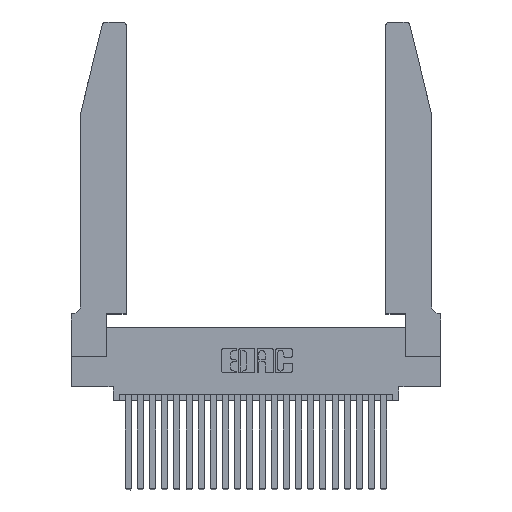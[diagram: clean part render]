
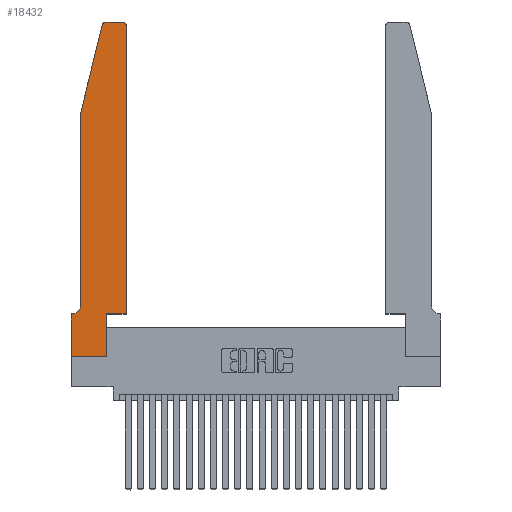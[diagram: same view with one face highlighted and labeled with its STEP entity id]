
A CAD part, top view. The second image highlights one B-rep face of the part: STEP entity #18432.
In plain terms, the highlighted planar face has unit normal (0, 0, 1).
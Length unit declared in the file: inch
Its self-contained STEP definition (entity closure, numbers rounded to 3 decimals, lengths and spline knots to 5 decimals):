
#32 = ORIENTED_EDGE ( 'NONE', *, *, #15384, .T. ) ;
#138 = CARTESIAN_POINT ( 'NONE',  ( 0., 0., 0.37 ) ) ;
#233 = ORIENTED_EDGE ( 'NONE', *, *, #24599, .T. ) ;
#419 = FACE_OUTER_BOUND ( 'NONE', #2256, .T. ) ;
#692 = DIRECTION ( 'NONE',  ( 0., 0., 1. ) ) ;
#938 = CARTESIAN_POINT ( 'NONE',  ( 0.0055, 0.42, 0.37 ) ) ;
#940 = PLANE ( 'NONE',  #18085 ) ;
#1878 = VERTEX_POINT ( 'NONE', #2045 ) ;
#2045 = CARTESIAN_POINT ( 'NONE',  ( 0., 0.35, 0.37 ) ) ;
#2124 = CIRCLE ( 'NONE', #16406, 0.07 ) ;
#2256 = EDGE_LOOP ( 'NONE', ( #233, #3412, #4674, #10498, #32, #19067, #16034, #11661, #19943, #14361, #12221, #11791 ) ) ;
#2813 = DIRECTION ( 'NONE',  ( 1., 0., 0. ) ) ;
#2917 = CARTESIAN_POINT ( 'NONE',  ( 0.2605, 2.75, 0.37 ) ) ;
#2941 = DIRECTION ( 'NONE',  ( 0., 0., 1. ) ) ;
#3209 = VERTEX_POINT ( 'NONE', #20163 ) ;
#3412 = ORIENTED_EDGE ( 'NONE', *, *, #7512, .T. ) ;
#4067 = LINE ( 'NONE', #9989, #20825 ) ;
#4369 = EDGE_CURVE ( 'NONE', #21793, #22872, #14482, .T. ) ;
#4428 = CARTESIAN_POINT ( 'NONE',  ( 0., 0.35, 0.37 ) ) ;
#4674 = ORIENTED_EDGE ( 'NONE', *, *, #23404, .T. ) ;
#4711 = AXIS2_PLACEMENT_3D ( 'NONE', #9152, #7432, #2813 ) ;
#5055 = CARTESIAN_POINT ( 'NONE',  ( 0.25487, 2.72718, 0.37 ) ) ;
#5305 = VERTEX_POINT ( 'NONE', #16759 ) ;
#5505 = LINE ( 'NONE', #2917, #9358 ) ;
#6192 = CARTESIAN_POINT ( 'NONE',  ( 0., 0., 0.37 ) ) ;
#6398 = VERTEX_POINT ( 'NONE', #5055 ) ;
#6475 = VECTOR ( 'NONE', #11939, 39.37008 ) ;
#6639 = CIRCLE ( 'NONE', #4711, 0.03 ) ;
#6866 = CARTESIAN_POINT ( 'NONE',  ( 0.0755, 0.42, 0.37 ) ) ;
#7374 = LINE ( 'NONE', #9487, #13313 ) ;
#7432 = DIRECTION ( 'NONE',  ( 0., 0., 1. ) ) ;
#7512 = EDGE_CURVE ( 'NONE', #3209, #6398, #7634, .T. ) ;
#7634 = CIRCLE ( 'NONE', #19590, 0.03 ) ;
#7831 = CARTESIAN_POINT ( 'NONE',  ( 0.0055, 0.35, 0.37 ) ) ;
#8262 = LINE ( 'NONE', #6192, #6475 ) ;
#8368 = CARTESIAN_POINT ( 'NONE',  ( 0.4505, 0.35, 0.37 ) ) ;
#8622 = CARTESIAN_POINT ( 'NONE',  ( 0.0755, 0.35, 0.37 ) ) ;
#8770 = DIRECTION ( 'NONE',  ( 1., 0., 0. ) ) ;
#8927 = CARTESIAN_POINT ( 'NONE',  ( 0., 0., 0.37 ) ) ;
#9152 = CARTESIAN_POINT ( 'NONE',  ( 0.4205, 2.72, 0.37 ) ) ;
#9326 = VECTOR ( 'NONE', #23130, 39.37008 ) ;
#9358 = VECTOR ( 'NONE', #16198, 39.37008 ) ;
#9365 = LINE ( 'NONE', #8622, #21090 ) ;
#9487 = CARTESIAN_POINT ( 'NONE',  ( 0.2865, 0.35, 0.37 ) ) ;
#9989 = CARTESIAN_POINT ( 'NONE',  ( 0.0755, 2., 0.37 ) ) ;
#10031 = LINE ( 'NONE', #8927, #22606 ) ;
#10269 = VECTOR ( 'NONE', #20962, 39.37008 ) ;
#10498 = ORIENTED_EDGE ( 'NONE', *, *, #4369, .T. ) ;
#11661 = ORIENTED_EDGE ( 'NONE', *, *, #22650, .T. ) ;
#11791 = ORIENTED_EDGE ( 'NONE', *, *, #13497, .T. ) ;
#11823 = EDGE_CURVE ( 'NONE', #5305, #22016, #21979, .T. ) ;
#11939 = DIRECTION ( 'NONE',  ( 1., 0., 0. ) ) ;
#12073 = DIRECTION ( 'NONE',  ( -1., 0., 0. ) ) ;
#12093 = CARTESIAN_POINT ( 'NONE',  ( 0.2865, 0., 0.37 ) ) ;
#12150 = DIRECTION ( 'NONE',  ( 1., 0., 0. ) ) ;
#12221 = ORIENTED_EDGE ( 'NONE', *, *, #18316, .T. ) ;
#12268 = EDGE_CURVE ( 'NONE', #16895, #1878, #9365, .T. ) ;
#12414 = CARTESIAN_POINT ( 'NONE',  ( 0.4505, 2.72, 0.37 ) ) ;
#12465 = DIRECTION ( 'NONE',  ( -1., 0., 0. ) ) ;
#13313 = VECTOR ( 'NONE', #15197, 39.37008 ) ;
#13497 = EDGE_CURVE ( 'NONE', #15955, #16582, #6639, .T. ) ;
#13506 = DIRECTION ( 'NONE',  ( 1., 0., 0. ) ) ;
#13640 = CARTESIAN_POINT ( 'NONE',  ( 0.0755, 2., 0.37 ) ) ;
#13845 = DIRECTION ( 'NONE',  ( -0.239, -0.971, 0. ) ) ;
#14361 = ORIENTED_EDGE ( 'NONE', *, *, #11823, .T. ) ;
#14482 = LINE ( 'NONE', #13640, #10269 ) ;
#15079 = CARTESIAN_POINT ( 'NONE',  ( 0.0755, 2., 0.37 ) ) ;
#15197 = DIRECTION ( 'NONE',  ( 0., 1., 0. ) ) ;
#15384 = EDGE_CURVE ( 'NONE', #22872, #16895, #2124, .T. ) ;
#15689 = VECTOR ( 'NONE', #13506, 39.37008 ) ;
#15864 = DIRECTION ( 'NONE',  ( 0., 0., -1. ) ) ;
#15955 = VERTEX_POINT ( 'NONE', #12414 ) ;
#16034 = ORIENTED_EDGE ( 'NONE', *, *, #22933, .T. ) ;
#16198 = DIRECTION ( 'NONE',  ( -1., 0., 0. ) ) ;
#16406 = AXIS2_PLACEMENT_3D ( 'NONE', #938, #15864, #12073 ) ;
#16582 = VERTEX_POINT ( 'NONE', #18477 ) ;
#16759 = CARTESIAN_POINT ( 'NONE',  ( 0.2865, 0.35, 0.37 ) ) ;
#16895 = VERTEX_POINT ( 'NONE', #7831 ) ;
#17727 = LINE ( 'NONE', #21392, #9326 ) ;
#18085 = AXIS2_PLACEMENT_3D ( 'NONE', #4428, #692, #12150 ) ;
#18316 = EDGE_CURVE ( 'NONE', #22016, #15955, #17727, .T. ) ;
#18432 = ADVANCED_FACE ( 'NONE', ( #419 ), #940, .T. ) ;
#18477 = CARTESIAN_POINT ( 'NONE',  ( 0.4205, 2.75, 0.37 ) ) ;
#19067 = ORIENTED_EDGE ( 'NONE', *, *, #12268, .T. ) ;
#19590 = AXIS2_PLACEMENT_3D ( 'NONE', #23812, #2941, #8770 ) ;
#19943 = ORIENTED_EDGE ( 'NONE', *, *, #23127, .T. ) ;
#20163 = CARTESIAN_POINT ( 'NONE',  ( 0.284, 2.75, 0.37 ) ) ;
#20603 = VERTEX_POINT ( 'NONE', #138 ) ;
#20657 = DIRECTION ( 'NONE',  ( 0., -1., 0. ) ) ;
#20825 = VECTOR ( 'NONE', #13845, 39.37008 ) ;
#20962 = DIRECTION ( 'NONE',  ( 0., -1., 0. ) ) ;
#21090 = VECTOR ( 'NONE', #12465, 39.37008 ) ;
#21295 = CARTESIAN_POINT ( 'NONE',  ( 0.4505, 0.35, 0.37 ) ) ;
#21392 = CARTESIAN_POINT ( 'NONE',  ( 0.4505, 0.35, 0.37 ) ) ;
#21793 = VERTEX_POINT ( 'NONE', #15079 ) ;
#21979 = LINE ( 'NONE', #21295, #15689 ) ;
#22016 = VERTEX_POINT ( 'NONE', #8368 ) ;
#22606 = VECTOR ( 'NONE', #20657, 39.37008 ) ;
#22650 = EDGE_CURVE ( 'NONE', #20603, #24513, #8262, .T. ) ;
#22872 = VERTEX_POINT ( 'NONE', #6866 ) ;
#22933 = EDGE_CURVE ( 'NONE', #1878, #20603, #10031, .T. ) ;
#23127 = EDGE_CURVE ( 'NONE', #24513, #5305, #7374, .T. ) ;
#23130 = DIRECTION ( 'NONE',  ( 0., 1., 0. ) ) ;
#23404 = EDGE_CURVE ( 'NONE', #6398, #21793, #4067, .T. ) ;
#23812 = CARTESIAN_POINT ( 'NONE',  ( 0.284, 2.72, 0.37 ) ) ;
#24513 = VERTEX_POINT ( 'NONE', #12093 ) ;
#24599 = EDGE_CURVE ( 'NONE', #16582, #3209, #5505, .T. ) ;
